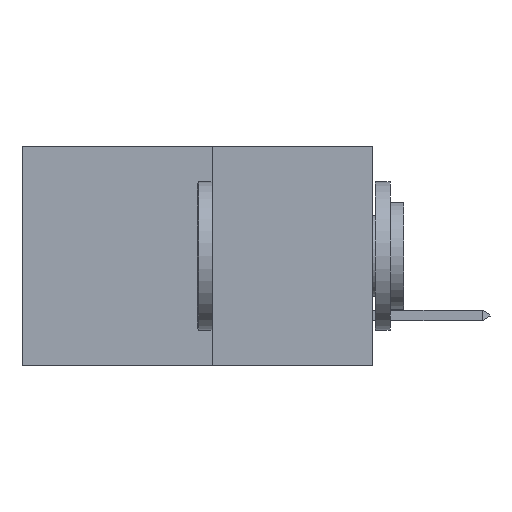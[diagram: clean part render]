
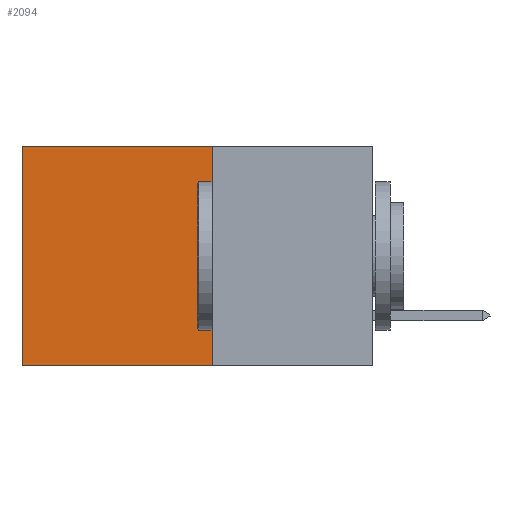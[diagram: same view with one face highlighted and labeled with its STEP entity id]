
A CAD part, left-side view. The second image highlights one B-rep face of the part: STEP entity #2094.
In plain terms, the highlighted planar face has unit normal (-1, 0, 0).
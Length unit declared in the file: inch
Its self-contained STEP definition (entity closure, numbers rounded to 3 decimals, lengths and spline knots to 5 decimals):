
#149 = CARTESIAN_POINT ( 'NONE',  ( 0.277, 0.27, -0.37 ) ) ;
#159 = LINE ( 'NONE', #8510, #17901 ) ;
#528 = VERTEX_POINT ( 'NONE', #13849 ) ;
#816 = VERTEX_POINT ( 'NONE', #12310 ) ;
#1778 = EDGE_CURVE ( 'NONE', #528, #3917, #159, .T. ) ;
#2094 = ADVANCED_FACE ( 'NONE', ( #16441 ), #14784, .F. ) ;
#2242 = VERTEX_POINT ( 'NONE', #3735 ) ;
#2386 = ORIENTED_EDGE ( 'NONE', *, *, #4471, .T. ) ;
#2392 = LINE ( 'NONE', #149, #13210 ) ;
#2632 = CARTESIAN_POINT ( 'NONE',  ( 0.277, 0.27, -0.37 ) ) ;
#2739 = ORIENTED_EDGE ( 'NONE', *, *, #13821, .F. ) ;
#3735 = CARTESIAN_POINT ( 'NONE',  ( 0.277, 0.27, 0. ) ) ;
#3917 = VERTEX_POINT ( 'NONE', #12385 ) ;
#4015 = DIRECTION ( 'NONE',  ( 0., 1., 0. ) ) ;
#4471 = EDGE_CURVE ( 'NONE', #2242, #528, #17759, .T. ) ;
#5061 = LINE ( 'NONE', #2632, #8363 ) ;
#6948 = VECTOR ( 'NONE', #9306, 39.37008 ) ;
#8091 = EDGE_CURVE ( 'NONE', #816, #3917, #5061, .T. ) ;
#8206 = DIRECTION ( 'NONE',  ( 0., 0., -1. ) ) ;
#8363 = VECTOR ( 'NONE', #4015, 39.37008 ) ;
#8510 = CARTESIAN_POINT ( 'NONE',  ( 0.277, 0.59, -0.37 ) ) ;
#9306 = DIRECTION ( 'NONE',  ( 0., 1., 0. ) ) ;
#10819 = CARTESIAN_POINT ( 'NONE',  ( 0.277, 0.27, 0. ) ) ;
#11977 = ORIENTED_EDGE ( 'NONE', *, *, #8091, .F. ) ;
#12310 = CARTESIAN_POINT ( 'NONE',  ( 0.277, 0.27, -0.37 ) ) ;
#12385 = CARTESIAN_POINT ( 'NONE',  ( 0.277, 0.59, -0.37 ) ) ;
#13210 = VECTOR ( 'NONE', #15676, 39.37008 ) ;
#13821 = EDGE_CURVE ( 'NONE', #2242, #816, #2392, .T. ) ;
#13849 = CARTESIAN_POINT ( 'NONE',  ( 0.277, 0.59, 0. ) ) ;
#14460 = EDGE_LOOP ( 'NONE', ( #18030, #11977, #2739, #2386 ) ) ;
#14634 = DIRECTION ( 'NONE',  ( 0., 0., -1. ) ) ;
#14705 = DIRECTION ( 'NONE',  ( 1., 0., 0. ) ) ;
#14784 = PLANE ( 'NONE',  #16983 ) ;
#14938 = CARTESIAN_POINT ( 'NONE',  ( 0.277, 0.27, -0.37 ) ) ;
#15676 = DIRECTION ( 'NONE',  ( 0., 0., -1. ) ) ;
#16441 = FACE_OUTER_BOUND ( 'NONE', #14460, .T. ) ;
#16983 = AXIS2_PLACEMENT_3D ( 'NONE', #14938, #14705, #14634 ) ;
#17759 = LINE ( 'NONE', #10819, #6948 ) ;
#17901 = VECTOR ( 'NONE', #8206, 39.37008 ) ;
#18030 = ORIENTED_EDGE ( 'NONE', *, *, #1778, .T. ) ;
